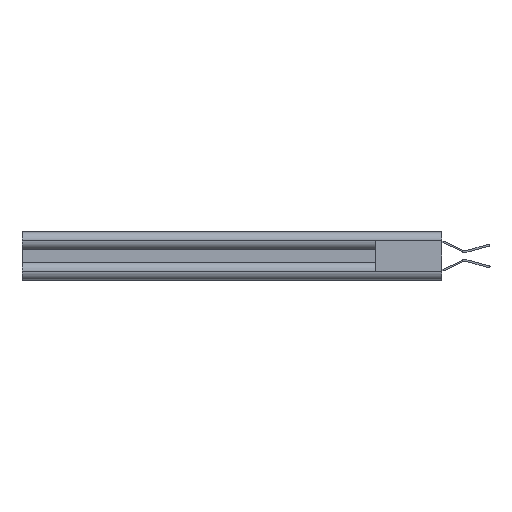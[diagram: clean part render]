
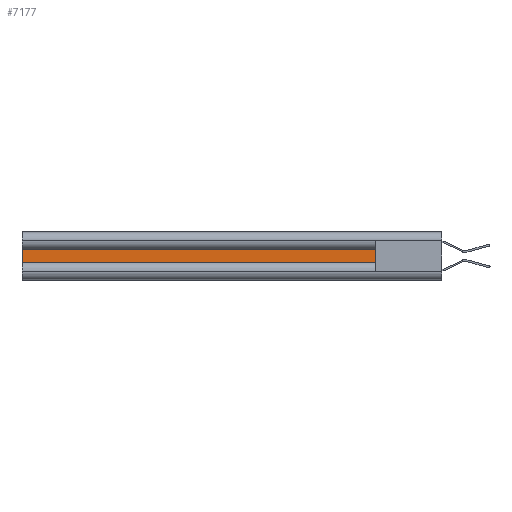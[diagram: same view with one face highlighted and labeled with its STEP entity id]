
A CAD part, left-side view. The second image highlights one B-rep face of the part: STEP entity #7177.
In plain terms, the highlighted planar face has unit normal (-1, 0, 0).
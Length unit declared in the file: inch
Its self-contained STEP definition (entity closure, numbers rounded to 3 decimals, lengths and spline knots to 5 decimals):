
#948 = DIRECTION ( 'NONE',  ( 0., 1., 0. ) ) ;
#1371 = LINE ( 'NONE', #1419, #10100 ) ;
#1419 = CARTESIAN_POINT ( 'NONE',  ( 0.044, 0.473, -0.0465 ) ) ;
#1931 = CARTESIAN_POINT ( 'NONE',  ( 0.044, 3., -0.0465 ) ) ;
#2366 = CARTESIAN_POINT ( 'NONE',  ( 0.044, 0.473, 0.0465 ) ) ;
#3340 = DIRECTION ( 'NONE',  ( 0., 1., 0. ) ) ;
#3611 = CARTESIAN_POINT ( 'NONE',  ( 0.044, 0.37012, -0.0465 ) ) ;
#3880 = LINE ( 'NONE', #1931, #12536 ) ;
#5390 = DIRECTION ( 'NONE',  ( 0., 0., -1. ) ) ;
#6346 = VECTOR ( 'NONE', #3340, 39.37008 ) ;
#6883 = CARTESIAN_POINT ( 'NONE',  ( 0.044, 3., -0.0465 ) ) ;
#7177 = ADVANCED_FACE ( 'NONE', ( #8862 ), #13908, .F. ) ;
#7201 = DIRECTION ( 'NONE',  ( 0., 0., -1. ) ) ;
#8124 = VECTOR ( 'NONE', #948, 39.37008 ) ;
#8356 = EDGE_CURVE ( 'NONE', #19038, #10490, #10957, .T. ) ;
#8862 = FACE_OUTER_BOUND ( 'NONE', #12055, .T. ) ;
#9328 = ORIENTED_EDGE ( 'NONE', *, *, #8356, .F. ) ;
#9659 = CARTESIAN_POINT ( 'NONE',  ( 0.044, 0.37012, 0.0465 ) ) ;
#10100 = VECTOR ( 'NONE', #18445, 39.37008 ) ;
#10124 = AXIS2_PLACEMENT_3D ( 'NONE', #3611, #15565, #5390 ) ;
#10490 = VERTEX_POINT ( 'NONE', #6883 ) ;
#10542 = CARTESIAN_POINT ( 'NONE',  ( 0.044, 0.473, -0.0465 ) ) ;
#10957 = LINE ( 'NONE', #21876, #6346 ) ;
#11346 = VERTEX_POINT ( 'NONE', #17645 ) ;
#12055 = EDGE_LOOP ( 'NONE', ( #12204, #18306, #9328, #13102 ) ) ;
#12204 = ORIENTED_EDGE ( 'NONE', *, *, #20873, .T. ) ;
#12536 = VECTOR ( 'NONE', #7201, 39.37008 ) ;
#12549 = EDGE_CURVE ( 'NONE', #11346, #10490, #3880, .T. ) ;
#13102 = ORIENTED_EDGE ( 'NONE', *, *, #13616, .F. ) ;
#13616 = EDGE_CURVE ( 'NONE', #14442, #19038, #1371, .T. ) ;
#13908 = PLANE ( 'NONE',  #10124 ) ;
#14442 = VERTEX_POINT ( 'NONE', #2366 ) ;
#15565 = DIRECTION ( 'NONE',  ( 1., 0., 0. ) ) ;
#17645 = CARTESIAN_POINT ( 'NONE',  ( 0.044, 3., 0.0465 ) ) ;
#18306 = ORIENTED_EDGE ( 'NONE', *, *, #12549, .T. ) ;
#18445 = DIRECTION ( 'NONE',  ( 0., 0., -1. ) ) ;
#19038 = VERTEX_POINT ( 'NONE', #10542 ) ;
#20873 = EDGE_CURVE ( 'NONE', #14442, #11346, #21413, .T. ) ;
#21413 = LINE ( 'NONE', #9659, #8124 ) ;
#21876 = CARTESIAN_POINT ( 'NONE',  ( 0.044, 0.37012, -0.0465 ) ) ;
